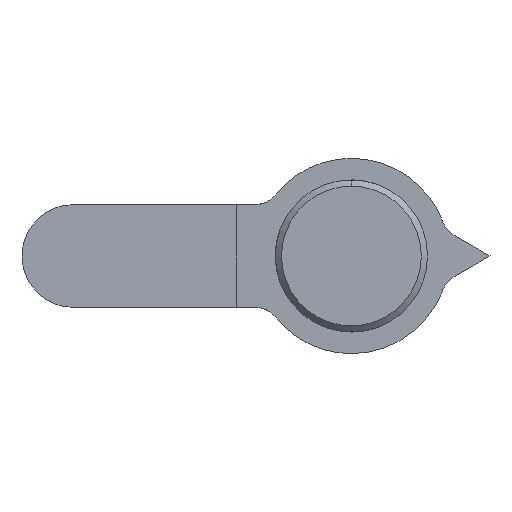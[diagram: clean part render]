
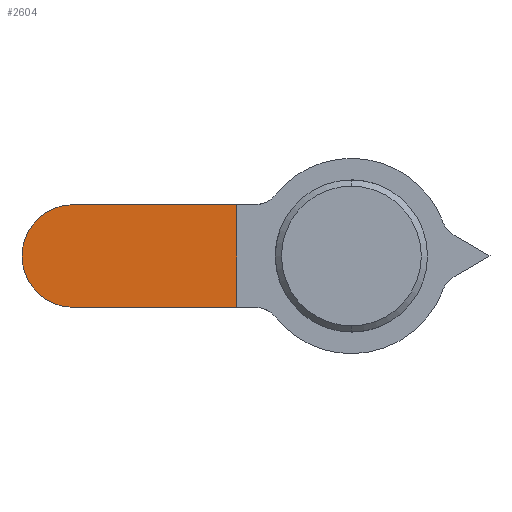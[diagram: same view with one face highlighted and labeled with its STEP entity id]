
A CAD part, front view. The second image highlights one B-rep face of the part: STEP entity #2604.
In plain terms, the highlighted planar face has unit normal (0, -1, 0).
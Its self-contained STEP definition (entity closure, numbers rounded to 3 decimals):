
#238 = CARTESIAN_POINT ( 'NONE',  ( -7.125, 24.333, 3.188 ) ) ;
#310 = ORIENTED_EDGE ( 'NONE', *, *, #2769, .T. ) ;
#312 = VECTOR ( 'NONE', #2962, 1000. ) ;
#492 = CARTESIAN_POINT ( 'NONE',  ( -7.125, 24.333, 3.188 ) ) ;
#586 = PLANE ( 'NONE',  #4435 ) ;
#597 = VERTEX_POINT ( 'NONE', #238 ) ;
#829 = LINE ( 'NONE', #492, #312 ) ;
#1144 = EDGE_LOOP ( 'NONE', ( #2522, #1976, #310, #4472 ) ) ;
#1200 = DIRECTION ( 'NONE',  ( 0., 0., 1. ) ) ;
#1478 = EDGE_CURVE ( 'NONE', #3879, #4278, #3529, .T. ) ;
#1672 = FACE_OUTER_BOUND ( 'NONE', #1144, .T. ) ;
#1927 = LINE ( 'NONE', #2546, #3002 ) ;
#1975 = DIRECTION ( 'NONE',  ( 0., 1., 0. ) ) ;
#1976 = ORIENTED_EDGE ( 'NONE', *, *, #3162, .T. ) ;
#2522 = ORIENTED_EDGE ( 'NONE', *, *, #3784, .T. ) ;
#2546 = CARTESIAN_POINT ( 'NONE',  ( -7.125, 24.333, -3.188 ) ) ;
#2604 = ADVANCED_FACE ( 'NONE', ( #1672 ), #586, .F. ) ;
#2700 = CARTESIAN_POINT ( 'NONE',  ( -27.163, 24.333, -10.858 ) ) ;
#2769 = EDGE_CURVE ( 'NONE', #597, #3879, #829, .T. ) ;
#2962 = DIRECTION ( 'NONE',  ( -1., 0., 0. ) ) ;
#3002 = VECTOR ( 'NONE', #3310, 1000. ) ;
#3048 = CARTESIAN_POINT ( 'NONE',  ( -17.247, 24.333, -3.188 ) ) ;
#3091 = DIRECTION ( 'NONE',  ( 1., 0., 0. ) ) ;
#3144 = VECTOR ( 'NONE', #3091, 1000. ) ;
#3162 = EDGE_CURVE ( 'NONE', #3173, #597, #1927, .T. ) ;
#3173 = VERTEX_POINT ( 'NONE', #3915 ) ;
#3310 = DIRECTION ( 'NONE',  ( 0., 0., 1. ) ) ;
#3431 = LINE ( 'NONE', #4198, #3144 ) ;
#3529 = CIRCLE ( 'NONE', #4458, 3.188 ) ;
#3537 = DIRECTION ( 'NONE',  ( 0., -1., 0. ) ) ;
#3634 = CARTESIAN_POINT ( 'NONE',  ( -17.247, 24.333, 3.188 ) ) ;
#3784 = EDGE_CURVE ( 'NONE', #4278, #3173, #3431, .T. ) ;
#3879 = VERTEX_POINT ( 'NONE', #3634 ) ;
#3895 = CARTESIAN_POINT ( 'NONE',  ( -17.247, 24.333, 0. ) ) ;
#3915 = CARTESIAN_POINT ( 'NONE',  ( -7.125, 24.333, -3.188 ) ) ;
#4198 = CARTESIAN_POINT ( 'NONE',  ( -17.247, 24.333, -3.188 ) ) ;
#4278 = VERTEX_POINT ( 'NONE', #3048 ) ;
#4393 = DIRECTION ( 'NONE',  ( 1., 0., 0. ) ) ;
#4435 = AXIS2_PLACEMENT_3D ( 'NONE', #2700, #1975, #4393 ) ;
#4458 = AXIS2_PLACEMENT_3D ( 'NONE', #3895, #3537, #1200 ) ;
#4472 = ORIENTED_EDGE ( 'NONE', *, *, #1478, .T. ) ;
